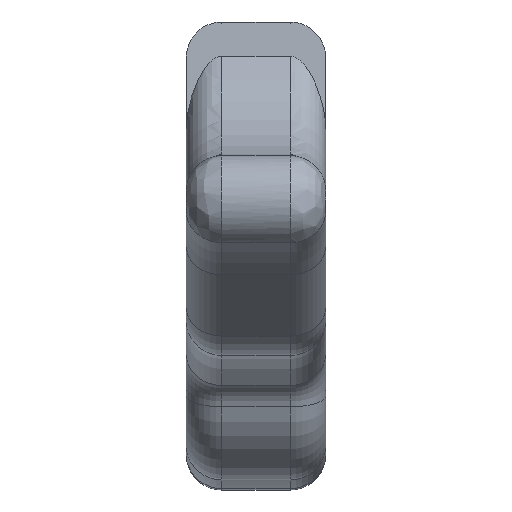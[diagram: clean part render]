
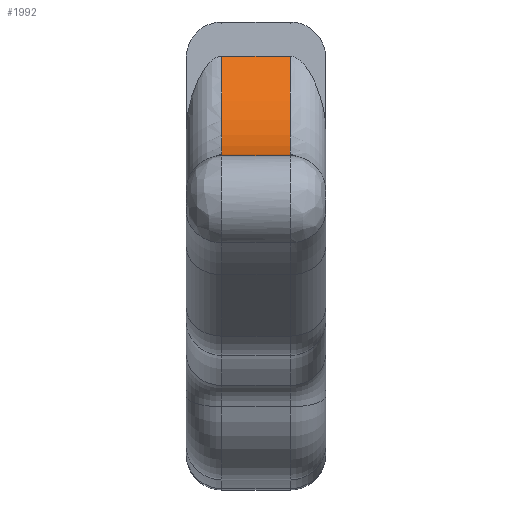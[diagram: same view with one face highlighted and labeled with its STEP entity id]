
A CAD part, front view. The second image highlights one B-rep face of the part: STEP entity #1992.
In plain terms, the highlighted cylindrical face has radius 12.652 mm (diameter 25.304 mm), a partial arc.
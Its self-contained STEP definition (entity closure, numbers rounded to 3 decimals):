
#29 = ORIENTED_EDGE ( 'NONE', *, *, #3453, .T. ) ;
#131 = CARTESIAN_POINT ( 'NONE',  ( -2.398, -9.625, 18.978 ) ) ;
#157 = CYLINDRICAL_SURFACE ( 'NONE', #1448, 12.652 ) ;
#274 = DIRECTION ( 'NONE',  ( 1., 0., 0. ) ) ;
#300 = AXIS2_PLACEMENT_3D ( 'NONE', #131, #2279, #444 ) ;
#444 = DIRECTION ( 'NONE',  ( 0., 0., -1. ) ) ;
#579 = EDGE_CURVE ( 'NONE', #2725, #2186, #2402, .T. ) ;
#712 = CARTESIAN_POINT ( 'NONE',  ( -26.013, -8.853, 6.35 ) ) ;
#951 = CARTESIAN_POINT ( 'NONE',  ( -2.398, 1.777, 13.495 ) ) ;
#1273 = ORIENTED_EDGE ( 'NONE', *, *, #2561, .F. ) ;
#1287 = CARTESIAN_POINT ( 'NONE',  ( 2.398, -9.625, 18.978 ) ) ;
#1414 = DIRECTION ( 'NONE',  ( 0., 0., -1. ) ) ;
#1448 = AXIS2_PLACEMENT_3D ( 'NONE', #2957, #3564, #1414 ) ;
#1592 = DIRECTION ( 'NONE',  ( 0., 0., -1. ) ) ;
#1604 = DIRECTION ( 'NONE',  ( 1., 0., 0. ) ) ;
#1659 = EDGE_CURVE ( 'NONE', #2705, #2725, #3982, .T. ) ;
#1752 = EDGE_LOOP ( 'NONE', ( #3878, #29, #1273, #1969 ) ) ;
#1780 = CARTESIAN_POINT ( 'NONE',  ( 2.398, 1.777, 13.495 ) ) ;
#1845 = VERTEX_POINT ( 'NONE', #1780 ) ;
#1969 = ORIENTED_EDGE ( 'NONE', *, *, #1659, .T. ) ;
#1992 = ADVANCED_FACE ( 'NONE', ( #2598 ), #157, .F. ) ;
#2110 = CARTESIAN_POINT ( 'NONE',  ( -26.013, 1.777, 13.495 ) ) ;
#2114 = CARTESIAN_POINT ( 'NONE',  ( 2.398, -8.853, 6.35 ) ) ;
#2186 = VERTEX_POINT ( 'NONE', #2114 ) ;
#2279 = DIRECTION ( 'NONE',  ( -1., 0., 0. ) ) ;
#2299 = CIRCLE ( 'NONE', #2845, 12.652 ) ;
#2402 = LINE ( 'NONE', #712, #3935 ) ;
#2561 = EDGE_CURVE ( 'NONE', #2705, #1845, #3601, .T. ) ;
#2598 = FACE_OUTER_BOUND ( 'NONE', #1752, .T. ) ;
#2705 = VERTEX_POINT ( 'NONE', #951 ) ;
#2725 = VERTEX_POINT ( 'NONE', #3098 ) ;
#2794 = VECTOR ( 'NONE', #274, 1000. ) ;
#2845 = AXIS2_PLACEMENT_3D ( 'NONE', #1287, #3432, #1592 ) ;
#2957 = CARTESIAN_POINT ( 'NONE',  ( -26.013, -9.625, 18.978 ) ) ;
#3098 = CARTESIAN_POINT ( 'NONE',  ( -2.398, -8.853, 6.35 ) ) ;
#3432 = DIRECTION ( 'NONE',  ( 1., 0., 0. ) ) ;
#3453 = EDGE_CURVE ( 'NONE', #2186, #1845, #2299, .T. ) ;
#3564 = DIRECTION ( 'NONE',  ( 1., 0., 0. ) ) ;
#3601 = LINE ( 'NONE', #2110, #2794 ) ;
#3878 = ORIENTED_EDGE ( 'NONE', *, *, #579, .T. ) ;
#3935 = VECTOR ( 'NONE', #1604, 1000. ) ;
#3982 = CIRCLE ( 'NONE', #300, 12.652 ) ;
